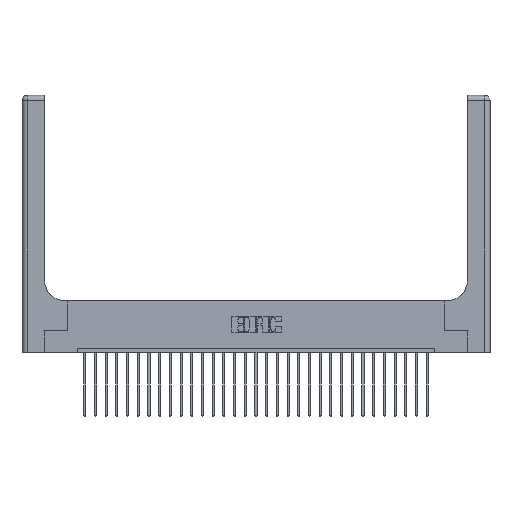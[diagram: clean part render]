
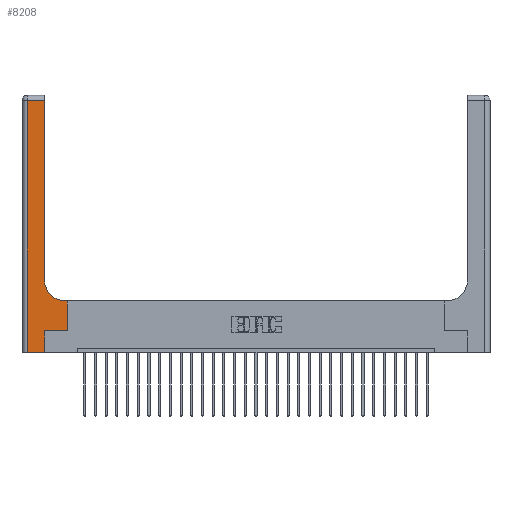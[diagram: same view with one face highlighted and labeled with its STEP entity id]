
A CAD part, top view. The second image highlights one B-rep face of the part: STEP entity #8208.
In plain terms, the highlighted planar face has unit normal (0, 0, 1).
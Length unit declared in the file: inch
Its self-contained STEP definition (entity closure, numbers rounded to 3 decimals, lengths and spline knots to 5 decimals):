
#62 = VERTEX_POINT ( 'NONE', #12211 ) ;
#616 = VECTOR ( 'NONE', #11902, 39.37008 ) ;
#1049 = CARTESIAN_POINT ( 'NONE',  ( 0.51, 0.85, 0.37 ) ) ;
#1564 = LINE ( 'NONE', #6047, #24955 ) ;
#1634 = DIRECTION ( 'NONE',  ( -1., 0., 0. ) ) ;
#1791 = CARTESIAN_POINT ( 'NONE',  ( 0., 3., 0.37 ) ) ;
#2083 = ORIENTED_EDGE ( 'NONE', *, *, #22478, .T. ) ;
#2551 = CARTESIAN_POINT ( 'NONE',  ( 0.26, 0.6, 0.37 ) ) ;
#2823 = EDGE_CURVE ( 'NONE', #13051, #8037, #21918, .T. ) ;
#3162 = LINE ( 'NONE', #17333, #13880 ) ;
#3962 = DIRECTION ( 'NONE',  ( 0., 0., -1. ) ) ;
#4033 = EDGE_CURVE ( 'NONE', #8037, #7975, #15355, .T. ) ;
#4325 = EDGE_CURVE ( 'NONE', #20853, #17728, #24114, .T. ) ;
#4557 = DIRECTION ( 'NONE',  ( 0., -1., 0. ) ) ;
#4799 = LINE ( 'NONE', #2551, #9663 ) ;
#5490 = EDGE_LOOP ( 'NONE', ( #15985, #12558, #10422, #2083, #21068, #8988, #17051, #11204, #17237 ) ) ;
#5729 = EDGE_CURVE ( 'NONE', #17734, #62, #6272, .T. ) ;
#6047 = CARTESIAN_POINT ( 'NONE',  ( 0., 2.94, 0.37 ) ) ;
#6085 = CARTESIAN_POINT ( 'NONE',  ( 0.265, 0., 0.37 ) ) ;
#6272 = LINE ( 'NONE', #21423, #23488 ) ;
#6494 = CARTESIAN_POINT ( 'NONE',  ( 0.26, 3., 0.37 ) ) ;
#6595 = CARTESIAN_POINT ( 'NONE',  ( 0.528, 0.6, 0.37 ) ) ;
#7760 = CARTESIAN_POINT ( 'NONE',  ( 0.265, 0.25, 0.37 ) ) ;
#7975 = VERTEX_POINT ( 'NONE', #19368 ) ;
#8037 = VERTEX_POINT ( 'NONE', #17979 ) ;
#8208 = ADVANCED_FACE ( 'NONE', ( #20460 ), #20453, .F. ) ;
#8686 = DIRECTION ( 'NONE',  ( 0., 1., 0. ) ) ;
#8988 = ORIENTED_EDGE ( 'NONE', *, *, #4325, .T. ) ;
#9471 = CARTESIAN_POINT ( 'NONE',  ( 0.265, 0.25, 0.37 ) ) ;
#9663 = VECTOR ( 'NONE', #11082, 39.37008 ) ;
#10422 = ORIENTED_EDGE ( 'NONE', *, *, #5729, .T. ) ;
#10504 = CARTESIAN_POINT ( 'NONE',  ( 0.51, 0.6, 0.37 ) ) ;
#10995 = LINE ( 'NONE', #22511, #616 ) ;
#11082 = DIRECTION ( 'NONE',  ( -1., 0., 0. ) ) ;
#11204 = ORIENTED_EDGE ( 'NONE', *, *, #15321, .T. ) ;
#11211 = DIRECTION ( 'NONE',  ( 0., 1., 0. ) ) ;
#11291 = DIRECTION ( 'NONE',  ( 1., 0., 0. ) ) ;
#11563 = DIRECTION ( 'NONE',  ( 0., 0., -1. ) ) ;
#11902 = DIRECTION ( 'NONE',  ( 0., 1., 0. ) ) ;
#12211 = CARTESIAN_POINT ( 'NONE',  ( 0.06, 0., 0.37 ) ) ;
#12558 = ORIENTED_EDGE ( 'NONE', *, *, #16471, .T. ) ;
#13051 = VERTEX_POINT ( 'NONE', #10504 ) ;
#13880 = VECTOR ( 'NONE', #11211, 39.37008 ) ;
#14056 = VECTOR ( 'NONE', #22067, 39.37008 ) ;
#14196 = CARTESIAN_POINT ( 'NONE',  ( 0., 0., 0.37 ) ) ;
#15050 = VECTOR ( 'NONE', #8686, 39.37008 ) ;
#15321 = EDGE_CURVE ( 'NONE', #25267, #13051, #4799, .T. ) ;
#15355 = LINE ( 'NONE', #6494, #15050 ) ;
#15925 = EDGE_CURVE ( 'NONE', #18476, #20853, #10995, .T. ) ;
#15985 = ORIENTED_EDGE ( 'NONE', *, *, #4033, .T. ) ;
#16471 = EDGE_CURVE ( 'NONE', #7975, #17734, #1564, .T. ) ;
#16513 = AXIS2_PLACEMENT_3D ( 'NONE', #1791, #3962, #18339 ) ;
#17051 = ORIENTED_EDGE ( 'NONE', *, *, #21205, .T. ) ;
#17237 = ORIENTED_EDGE ( 'NONE', *, *, #2823, .T. ) ;
#17333 = CARTESIAN_POINT ( 'NONE',  ( 0.528, 0.25, 0.37 ) ) ;
#17728 = VERTEX_POINT ( 'NONE', #26036 ) ;
#17734 = VERTEX_POINT ( 'NONE', #19912 ) ;
#17979 = CARTESIAN_POINT ( 'NONE',  ( 0.26, 0.85, 0.37 ) ) ;
#18339 = DIRECTION ( 'NONE',  ( -1., 0., 0. ) ) ;
#18476 = VERTEX_POINT ( 'NONE', #6085 ) ;
#18706 = DIRECTION ( 'NONE',  ( 1., 0., 0. ) ) ;
#19349 = AXIS2_PLACEMENT_3D ( 'NONE', #1049, #11563, #11291 ) ;
#19368 = CARTESIAN_POINT ( 'NONE',  ( 0.26, 2.94, 0.37 ) ) ;
#19912 = CARTESIAN_POINT ( 'NONE',  ( 0.06, 2.94, 0.37 ) ) ;
#20453 = PLANE ( 'NONE',  #16513 ) ;
#20460 = FACE_OUTER_BOUND ( 'NONE', #5490, .T. ) ;
#20853 = VERTEX_POINT ( 'NONE', #7760 ) ;
#21068 = ORIENTED_EDGE ( 'NONE', *, *, #15925, .T. ) ;
#21205 = EDGE_CURVE ( 'NONE', #17728, #25267, #3162, .T. ) ;
#21281 = VECTOR ( 'NONE', #18706, 39.37008 ) ;
#21423 = CARTESIAN_POINT ( 'NONE',  ( 0.06, 3., 0.37 ) ) ;
#21918 = CIRCLE ( 'NONE', #19349, 0.25 ) ;
#22067 = DIRECTION ( 'NONE',  ( 1., 0., 0. ) ) ;
#22478 = EDGE_CURVE ( 'NONE', #62, #18476, #25518, .T. ) ;
#22511 = CARTESIAN_POINT ( 'NONE',  ( 0.265, 0., 0.37 ) ) ;
#23488 = VECTOR ( 'NONE', #4557, 39.37008 ) ;
#24114 = LINE ( 'NONE', #9471, #14056 ) ;
#24955 = VECTOR ( 'NONE', #1634, 39.37008 ) ;
#25267 = VERTEX_POINT ( 'NONE', #6595 ) ;
#25518 = LINE ( 'NONE', #14196, #21281 ) ;
#26036 = CARTESIAN_POINT ( 'NONE',  ( 0.528, 0.25, 0.37 ) ) ;
